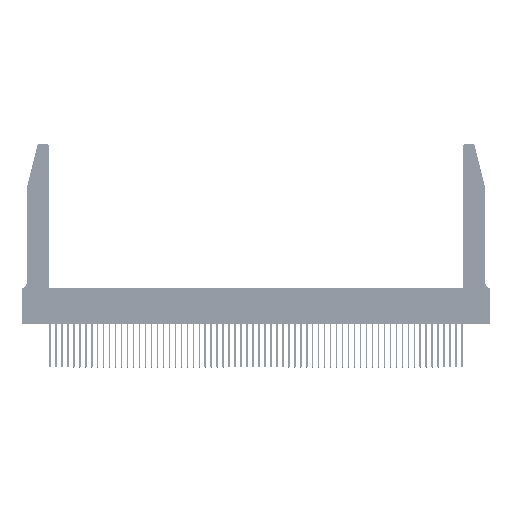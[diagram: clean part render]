
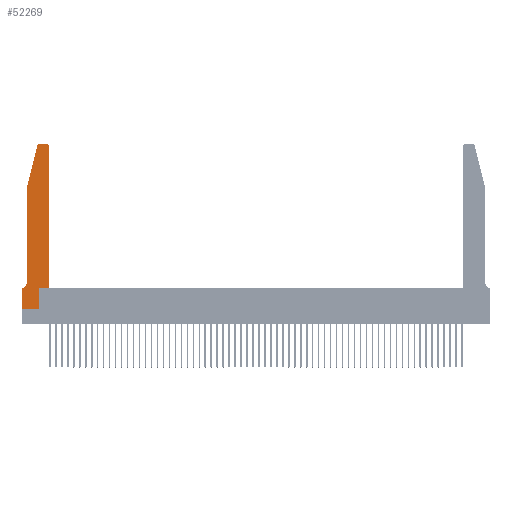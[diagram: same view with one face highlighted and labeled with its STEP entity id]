
A CAD part, top view. The second image highlights one B-rep face of the part: STEP entity #52269.
In plain terms, the highlighted planar face has unit normal (0, 0, 1).
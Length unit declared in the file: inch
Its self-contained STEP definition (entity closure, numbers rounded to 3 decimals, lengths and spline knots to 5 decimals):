
#614 = CARTESIAN_POINT ( 'NONE',  ( 0., 0.35, 0.37 ) ) ;
#1062 = CARTESIAN_POINT ( 'NONE',  ( 0.0755, 2., 0.37 ) ) ;
#1230 = LINE ( 'NONE', #45695, #45865 ) ;
#2194 = VERTEX_POINT ( 'NONE', #40451 ) ;
#2337 = VECTOR ( 'NONE', #29921, 39.37008 ) ;
#2982 = CIRCLE ( 'NONE', #47026, 0.03 ) ;
#3137 = FACE_OUTER_BOUND ( 'NONE', #47674, .T. ) ;
#3632 = EDGE_CURVE ( 'NONE', #28013, #36727, #50457, .T. ) ;
#3954 = DIRECTION ( 'NONE',  ( 1., 0., 0. ) ) ;
#4361 = DIRECTION ( 'NONE',  ( -0.239, -0.971, 0. ) ) ;
#4528 = ORIENTED_EDGE ( 'NONE', *, *, #15264, .T. ) ;
#4983 = DIRECTION ( 'NONE',  ( 1., 0., 0. ) ) ;
#6385 = LINE ( 'NONE', #17107, #2337 ) ;
#7784 = ORIENTED_EDGE ( 'NONE', *, *, #30351, .T. ) ;
#8799 = CARTESIAN_POINT ( 'NONE',  ( 0.284, 2.72, 0.37 ) ) ;
#9145 = DIRECTION ( 'NONE',  ( -1., 0., 0. ) ) ;
#10177 = ORIENTED_EDGE ( 'NONE', *, *, #48125, .T. ) ;
#11145 = VERTEX_POINT ( 'NONE', #14305 ) ;
#11367 = EDGE_CURVE ( 'NONE', #27803, #20672, #28812, .T. ) ;
#12379 = CARTESIAN_POINT ( 'NONE',  ( 0.2865, 0., 0.37 ) ) ;
#12415 = VECTOR ( 'NONE', #49364, 39.37008 ) ;
#13185 = DIRECTION ( 'NONE',  ( 1., 0., 0. ) ) ;
#13765 = AXIS2_PLACEMENT_3D ( 'NONE', #24131, #54221, #28447 ) ;
#14305 = CARTESIAN_POINT ( 'NONE',  ( 0.2865, 0.35, 0.37 ) ) ;
#14580 = CARTESIAN_POINT ( 'NONE',  ( 0., 0., 0.37 ) ) ;
#15264 = EDGE_CURVE ( 'NONE', #44946, #11145, #1230, .T. ) ;
#16094 = VECTOR ( 'NONE', #9145, 39.37008 ) ;
#16223 = EDGE_CURVE ( 'NONE', #2194, #21891, #45771, .T. ) ;
#17107 = CARTESIAN_POINT ( 'NONE',  ( 0., 0., 0.37 ) ) ;
#17250 = ORIENTED_EDGE ( 'NONE', *, *, #52237, .T. ) ;
#17263 = CARTESIAN_POINT ( 'NONE',  ( 0., 0., 0.37 ) ) ;
#17335 = VECTOR ( 'NONE', #45966, 39.37008 ) ;
#17544 = VECTOR ( 'NONE', #47385, 39.37008 ) ;
#19501 = CARTESIAN_POINT ( 'NONE',  ( 0.4505, 0.35, 0.37 ) ) ;
#20672 = VERTEX_POINT ( 'NONE', #52569 ) ;
#21891 = VERTEX_POINT ( 'NONE', #1062 ) ;
#22420 = VECTOR ( 'NONE', #49004, 39.37008 ) ;
#23412 = CARTESIAN_POINT ( 'NONE',  ( 0.4505, 0.35, 0.37 ) ) ;
#24131 = CARTESIAN_POINT ( 'NONE',  ( 0.0055, 0.42, 0.37 ) ) ;
#24240 = VECTOR ( 'NONE', #4361, 39.37008 ) ;
#25487 = ORIENTED_EDGE ( 'NONE', *, *, #45816, .T. ) ;
#25974 = CARTESIAN_POINT ( 'NONE',  ( 0.0755, 2., 0.37 ) ) ;
#26668 = VECTOR ( 'NONE', #49833, 39.37008 ) ;
#27803 = VERTEX_POINT ( 'NONE', #31635 ) ;
#28013 = VERTEX_POINT ( 'NONE', #48031 ) ;
#28025 = LINE ( 'NONE', #19501, #26668 ) ;
#28447 = DIRECTION ( 'NONE',  ( -1., 0., 0. ) ) ;
#28812 = LINE ( 'NONE', #41650, #17335 ) ;
#28862 = ORIENTED_EDGE ( 'NONE', *, *, #11367, .T. ) ;
#29012 = LINE ( 'NONE', #17263, #17544 ) ;
#29043 = VERTEX_POINT ( 'NONE', #33591 ) ;
#29890 = DIRECTION ( 'NONE',  ( 0., 0., 1. ) ) ;
#29921 = DIRECTION ( 'NONE',  ( 0., -1., 0. ) ) ;
#30228 = LINE ( 'NONE', #35044, #16094 ) ;
#30351 = EDGE_CURVE ( 'NONE', #44599, #51457, #6385, .T. ) ;
#30913 = DIRECTION ( 'NONE',  ( 0., 0., 1. ) ) ;
#31550 = EDGE_CURVE ( 'NONE', #20672, #2194, #53810, .T. ) ;
#31635 = CARTESIAN_POINT ( 'NONE',  ( 0.4205, 2.75, 0.37 ) ) ;
#33550 = ORIENTED_EDGE ( 'NONE', *, *, #16223, .T. ) ;
#33591 = CARTESIAN_POINT ( 'NONE',  ( 0.4505, 2.72, 0.37 ) ) ;
#35044 = CARTESIAN_POINT ( 'NONE',  ( 0.0755, 0.35, 0.37 ) ) ;
#35745 = ORIENTED_EDGE ( 'NONE', *, *, #31550, .T. ) ;
#35753 = ORIENTED_EDGE ( 'NONE', *, *, #44555, .T. ) ;
#35894 = CARTESIAN_POINT ( 'NONE',  ( 0.0055, 0.35, 0.37 ) ) ;
#36727 = VERTEX_POINT ( 'NONE', #35894 ) ;
#39064 = DIRECTION ( 'NONE',  ( 0., 0., 1. ) ) ;
#40451 = CARTESIAN_POINT ( 'NONE',  ( 0.25487, 2.72718, 0.37 ) ) ;
#41650 = CARTESIAN_POINT ( 'NONE',  ( 0.2605, 2.75, 0.37 ) ) ;
#42661 = EDGE_CURVE ( 'NONE', #11145, #55820, #28025, .T. ) ;
#42806 = AXIS2_PLACEMENT_3D ( 'NONE', #614, #30913, #4983 ) ;
#43724 = PLANE ( 'NONE',  #42806 ) ;
#44555 = EDGE_CURVE ( 'NONE', #21891, #28013, #55416, .T. ) ;
#44599 = VERTEX_POINT ( 'NONE', #44832 ) ;
#44631 = CARTESIAN_POINT ( 'NONE',  ( 0.0755, 2., 0.37 ) ) ;
#44832 = CARTESIAN_POINT ( 'NONE',  ( 0., 0.35, 0.37 ) ) ;
#44946 = VERTEX_POINT ( 'NONE', #12379 ) ;
#44997 = CARTESIAN_POINT ( 'NONE',  ( 0.4505, 0.35, 0.37 ) ) ;
#45695 = CARTESIAN_POINT ( 'NONE',  ( 0.2865, 0.35, 0.37 ) ) ;
#45771 = LINE ( 'NONE', #25974, #24240 ) ;
#45816 = EDGE_CURVE ( 'NONE', #51457, #44946, #29012, .T. ) ;
#45865 = VECTOR ( 'NONE', #50048, 39.37008 ) ;
#45966 = DIRECTION ( 'NONE',  ( -1., 0., 0. ) ) ;
#46492 = ORIENTED_EDGE ( 'NONE', *, *, #42661, .T. ) ;
#46841 = LINE ( 'NONE', #44997, #12415 ) ;
#47026 = AXIS2_PLACEMENT_3D ( 'NONE', #55681, #29890, #3954 ) ;
#47385 = DIRECTION ( 'NONE',  ( 1., 0., 0. ) ) ;
#47674 = EDGE_LOOP ( 'NONE', ( #28862, #35745, #33550, #35753, #48143, #17250, #7784, #25487, #4528, #46492, #48633, #10177 ) ) ;
#48031 = CARTESIAN_POINT ( 'NONE',  ( 0.0755, 0.42, 0.37 ) ) ;
#48125 = EDGE_CURVE ( 'NONE', #29043, #27803, #2982, .T. ) ;
#48143 = ORIENTED_EDGE ( 'NONE', *, *, #3632, .T. ) ;
#48633 = ORIENTED_EDGE ( 'NONE', *, *, #48772, .T. ) ;
#48772 = EDGE_CURVE ( 'NONE', #55820, #29043, #46841, .T. ) ;
#49004 = DIRECTION ( 'NONE',  ( 0., -1., 0. ) ) ;
#49364 = DIRECTION ( 'NONE',  ( 0., 1., 0. ) ) ;
#49833 = DIRECTION ( 'NONE',  ( 1., 0., 0. ) ) ;
#50048 = DIRECTION ( 'NONE',  ( 0., 1., 0. ) ) ;
#50457 = CIRCLE ( 'NONE', #13765, 0.07 ) ;
#51457 = VERTEX_POINT ( 'NONE', #14580 ) ;
#52237 = EDGE_CURVE ( 'NONE', #36727, #44599, #30228, .T. ) ;
#52269 = ADVANCED_FACE ( 'NONE', ( #3137 ), #43724, .T. ) ;
#52290 = AXIS2_PLACEMENT_3D ( 'NONE', #8799, #39064, #13185 ) ;
#52569 = CARTESIAN_POINT ( 'NONE',  ( 0.284, 2.75, 0.37 ) ) ;
#53810 = CIRCLE ( 'NONE', #52290, 0.03 ) ;
#54221 = DIRECTION ( 'NONE',  ( 0., 0., -1. ) ) ;
#55416 = LINE ( 'NONE', #44631, #22420 ) ;
#55681 = CARTESIAN_POINT ( 'NONE',  ( 0.4205, 2.72, 0.37 ) ) ;
#55820 = VERTEX_POINT ( 'NONE', #23412 ) ;
